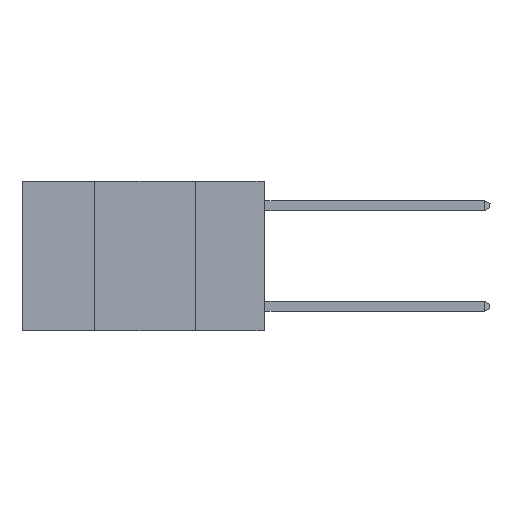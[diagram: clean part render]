
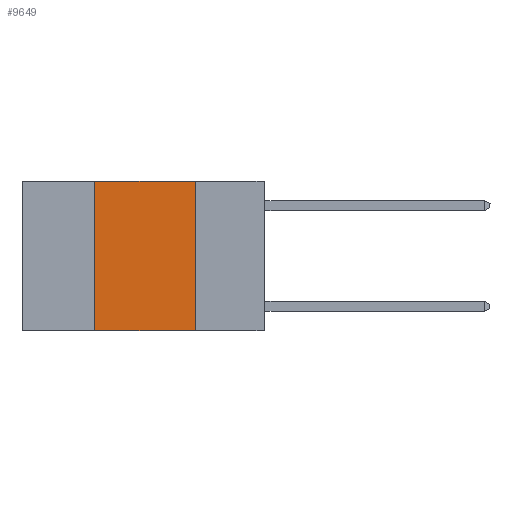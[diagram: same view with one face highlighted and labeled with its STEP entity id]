
A CAD part, left-side view. The second image highlights one B-rep face of the part: STEP entity #9649.
In plain terms, the highlighted planar face has unit normal (-1, 0, 0).
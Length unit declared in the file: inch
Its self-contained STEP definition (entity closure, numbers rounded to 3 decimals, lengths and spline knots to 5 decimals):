
#115 = LINE ( 'NONE', #3734, #13020 ) ;
#2417 = ORIENTED_EDGE ( 'NONE', *, *, #21280, .F. ) ;
#2480 = AXIS2_PLACEMENT_3D ( 'NONE', #5142, #16956, #19956 ) ;
#2712 = PLANE ( 'NONE',  #2480 ) ;
#3058 = VERTEX_POINT ( 'NONE', #20678 ) ;
#3734 = CARTESIAN_POINT ( 'NONE',  ( 0., 0.6, -0.37 ) ) ;
#4259 = VECTOR ( 'NONE', #16198, 39.37008 ) ;
#4981 = DIRECTION ( 'NONE',  ( 0., 0., 1. ) ) ;
#5142 = CARTESIAN_POINT ( 'NONE',  ( 0., 0.6, 0. ) ) ;
#5520 = EDGE_CURVE ( 'NONE', #3058, #17722, #10282, .T. ) ;
#5584 = ORIENTED_EDGE ( 'NONE', *, *, #7105, .F. ) ;
#6691 = VECTOR ( 'NONE', #8388, 39.37008 ) ;
#6747 = VECTOR ( 'NONE', #4981, 39.37008 ) ;
#7022 = LINE ( 'NONE', #17783, #4259 ) ;
#7105 = EDGE_CURVE ( 'NONE', #17494, #3058, #16683, .T. ) ;
#8209 = EDGE_LOOP ( 'NONE', ( #2417, #10488, #5584, #20436 ) ) ;
#8388 = DIRECTION ( 'NONE',  ( 0., -1., 0. ) ) ;
#8715 = CARTESIAN_POINT ( 'NONE',  ( 0., 0.42, -0.37 ) ) ;
#8930 = CARTESIAN_POINT ( 'NONE',  ( 0., 0.17, 0. ) ) ;
#9232 = VERTEX_POINT ( 'NONE', #10077 ) ;
#9649 = ADVANCED_FACE ( 'NONE', ( #13548 ), #2712, .F. ) ;
#10077 = CARTESIAN_POINT ( 'NONE',  ( 0., 0.17, -0.37 ) ) ;
#10282 = LINE ( 'NONE', #17209, #6691 ) ;
#10488 = ORIENTED_EDGE ( 'NONE', *, *, #5520, .F. ) ;
#10710 = EDGE_CURVE ( 'NONE', #17494, #9232, #115, .T. ) ;
#12000 = DIRECTION ( 'NONE',  ( 0., -1., 0. ) ) ;
#13020 = VECTOR ( 'NONE', #12000, 39.37008 ) ;
#13548 = FACE_OUTER_BOUND ( 'NONE', #8209, .T. ) ;
#16198 = DIRECTION ( 'NONE',  ( 0., 0., -1. ) ) ;
#16683 = LINE ( 'NONE', #22349, #6747 ) ;
#16956 = DIRECTION ( 'NONE',  ( 1., 0., 0. ) ) ;
#17209 = CARTESIAN_POINT ( 'NONE',  ( 0., 0.6, 0. ) ) ;
#17494 = VERTEX_POINT ( 'NONE', #8715 ) ;
#17722 = VERTEX_POINT ( 'NONE', #8930 ) ;
#17783 = CARTESIAN_POINT ( 'NONE',  ( 0., 0.17, 0. ) ) ;
#19956 = DIRECTION ( 'NONE',  ( 0., 0., -1. ) ) ;
#20436 = ORIENTED_EDGE ( 'NONE', *, *, #10710, .T. ) ;
#20678 = CARTESIAN_POINT ( 'NONE',  ( 0., 0.42, 0. ) ) ;
#21280 = EDGE_CURVE ( 'NONE', #17722, #9232, #7022, .T. ) ;
#22349 = CARTESIAN_POINT ( 'NONE',  ( 0., 0.42, 0. ) ) ;
